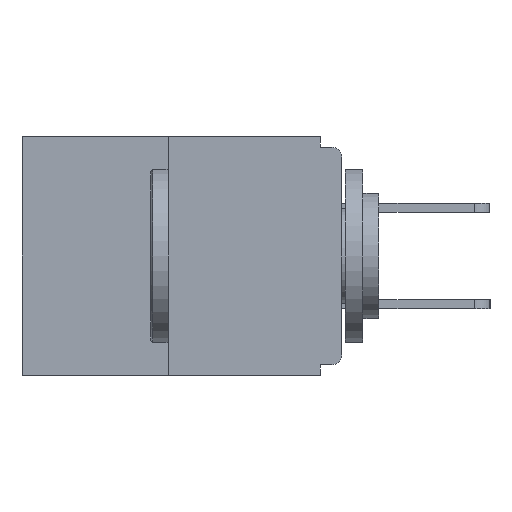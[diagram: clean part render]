
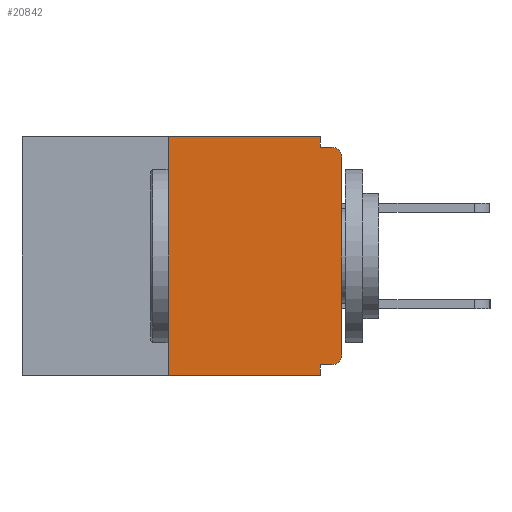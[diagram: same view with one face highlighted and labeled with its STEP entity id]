
A CAD part, left-side view. The second image highlights one B-rep face of the part: STEP entity #20842.
In plain terms, the highlighted planar face has unit normal (-1, 0, 0).
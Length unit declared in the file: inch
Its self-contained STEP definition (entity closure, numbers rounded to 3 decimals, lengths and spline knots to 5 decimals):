
#35 = VERTEX_POINT ( 'NONE', #1568 ) ;
#223 = CARTESIAN_POINT ( 'NONE',  ( 0., 0., 0. ) ) ;
#266 = DIRECTION ( 'NONE',  ( 0., 0., 1. ) ) ;
#528 = VECTOR ( 'NONE', #5872, 39.37008 ) ;
#721 = ORIENTED_EDGE ( 'NONE', *, *, #4216, .T. ) ;
#726 = VECTOR ( 'NONE', #266, 39.37008 ) ;
#1271 = CARTESIAN_POINT ( 'NONE',  ( 0., 0.031, -0.015 ) ) ;
#1568 = CARTESIAN_POINT ( 'NONE',  ( 0., 0.015, -0.015 ) ) ;
#2616 = ORIENTED_EDGE ( 'NONE', *, *, #19204, .T. ) ;
#2681 = EDGE_CURVE ( 'NONE', #5634, #35, #19461, .T. ) ;
#3198 = ORIENTED_EDGE ( 'NONE', *, *, #7958, .F. ) ;
#3575 = VERTEX_POINT ( 'NONE', #24287 ) ;
#4006 = EDGE_LOOP ( 'NONE', ( #14954, #20525, #4340, #3198, #5265, #721, #2616, #23189, #13043, #9560 ) ) ;
#4199 = CARTESIAN_POINT ( 'NONE',  ( 0., 0., -0.015 ) ) ;
#4216 = EDGE_CURVE ( 'NONE', #17066, #3575, #17351, .T. ) ;
#4247 = DIRECTION ( 'NONE',  ( -1., 0., 0. ) ) ;
#4340 = ORIENTED_EDGE ( 'NONE', *, *, #8797, .T. ) ;
#4409 = PLANE ( 'NONE',  #13137 ) ;
#4640 = LINE ( 'NONE', #4199, #528 ) ;
#4915 = CARTESIAN_POINT ( 'NONE',  ( 0., 0.25, 0. ) ) ;
#5029 = LINE ( 'NONE', #8013, #17426 ) ;
#5265 = ORIENTED_EDGE ( 'NONE', *, *, #10138, .F. ) ;
#5357 = LINE ( 'NONE', #17469, #25343 ) ;
#5634 = VERTEX_POINT ( 'NONE', #7228 ) ;
#5655 = VECTOR ( 'NONE', #16438, 39.37008 ) ;
#5872 = DIRECTION ( 'NONE',  ( 0., -1., 0. ) ) ;
#7049 = CARTESIAN_POINT ( 'NONE',  ( 0., 0.031, -0.328 ) ) ;
#7228 = CARTESIAN_POINT ( 'NONE',  ( 0., 0., -0.03 ) ) ;
#7535 = LINE ( 'NONE', #25013, #12930 ) ;
#7699 = CARTESIAN_POINT ( 'NONE',  ( 0., 0.25, -0.343 ) ) ;
#7958 = EDGE_CURVE ( 'NONE', #10662, #8174, #5357, .T. ) ;
#8013 = CARTESIAN_POINT ( 'NONE',  ( 0., 0., -0.328 ) ) ;
#8174 = VERTEX_POINT ( 'NONE', #10585 ) ;
#8677 = DIRECTION ( 'NONE',  ( 0., 0., -1. ) ) ;
#8797 = EDGE_CURVE ( 'NONE', #16553, #8174, #7535, .T. ) ;
#9279 = EDGE_CURVE ( 'NONE', #26026, #16123, #17357, .T. ) ;
#9560 = ORIENTED_EDGE ( 'NONE', *, *, #16487, .F. ) ;
#9629 = AXIS2_PLACEMENT_3D ( 'NONE', #12190, #4247, #18341 ) ;
#9908 = CARTESIAN_POINT ( 'NONE',  ( 0., 0.015, -0.03 ) ) ;
#10138 = EDGE_CURVE ( 'NONE', #17066, #10662, #5029, .T. ) ;
#10179 = DIRECTION ( 'NONE',  ( -1., 0., 0. ) ) ;
#10585 = CARTESIAN_POINT ( 'NONE',  ( 0., 0.031, -0.343 ) ) ;
#10662 = VERTEX_POINT ( 'NONE', #7049 ) ;
#11178 = LINE ( 'NONE', #20848, #24805 ) ;
#11510 = AXIS2_PLACEMENT_3D ( 'NONE', #9908, #10179, #16242 ) ;
#12183 = CARTESIAN_POINT ( 'NONE',  ( 0., 0.46, 0. ) ) ;
#12190 = CARTESIAN_POINT ( 'NONE',  ( 0., 0.015, -0.313 ) ) ;
#12930 = VECTOR ( 'NONE', #16897, 39.37008 ) ;
#13043 = ORIENTED_EDGE ( 'NONE', *, *, #20962, .F. ) ;
#13137 = AXIS2_PLACEMENT_3D ( 'NONE', #12183, #18588, #22471 ) ;
#13470 = DIRECTION ( 'NONE',  ( 0., -1., 0. ) ) ;
#13480 = EDGE_CURVE ( 'NONE', #16553, #26026, #16903, .T. ) ;
#13993 = DIRECTION ( 'NONE',  ( 0., 0., -1. ) ) ;
#14392 = VERTEX_POINT ( 'NONE', #1271 ) ;
#14954 = ORIENTED_EDGE ( 'NONE', *, *, #9279, .F. ) ;
#15310 = CARTESIAN_POINT ( 'NONE',  ( 0., 0.031, 0. ) ) ;
#16123 = VERTEX_POINT ( 'NONE', #15310 ) ;
#16242 = DIRECTION ( 'NONE',  ( 0., 0., -1. ) ) ;
#16438 = DIRECTION ( 'NONE',  ( 0., 0., 1. ) ) ;
#16487 = EDGE_CURVE ( 'NONE', #16123, #14392, #11178, .T. ) ;
#16553 = VERTEX_POINT ( 'NONE', #7699 ) ;
#16698 = FACE_OUTER_BOUND ( 'NONE', #4006, .T. ) ;
#16897 = DIRECTION ( 'NONE',  ( 0., -1., 0. ) ) ;
#16903 = LINE ( 'NONE', #20377, #726 ) ;
#17066 = VERTEX_POINT ( 'NONE', #25762 ) ;
#17351 = CIRCLE ( 'NONE', #9629, 0.015 ) ;
#17357 = LINE ( 'NONE', #25599, #24630 ) ;
#17426 = VECTOR ( 'NONE', #20443, 39.37008 ) ;
#17469 = CARTESIAN_POINT ( 'NONE',  ( 0., 0.031, -0.343 ) ) ;
#18341 = DIRECTION ( 'NONE',  ( 0., 0., -1. ) ) ;
#18588 = DIRECTION ( 'NONE',  ( 1., 0., 0. ) ) ;
#18664 = LINE ( 'NONE', #223, #5655 ) ;
#19204 = EDGE_CURVE ( 'NONE', #3575, #5634, #18664, .T. ) ;
#19461 = CIRCLE ( 'NONE', #11510, 0.015 ) ;
#20377 = CARTESIAN_POINT ( 'NONE',  ( 0., 0.25, 0. ) ) ;
#20443 = DIRECTION ( 'NONE',  ( 0., 1., 0. ) ) ;
#20525 = ORIENTED_EDGE ( 'NONE', *, *, #13480, .F. ) ;
#20842 = ADVANCED_FACE ( 'NONE', ( #16698 ), #4409, .F. ) ;
#20848 = CARTESIAN_POINT ( 'NONE',  ( 0., 0.031, 0. ) ) ;
#20962 = EDGE_CURVE ( 'NONE', #14392, #35, #4640, .T. ) ;
#22471 = DIRECTION ( 'NONE',  ( 0., 0., -1. ) ) ;
#23189 = ORIENTED_EDGE ( 'NONE', *, *, #2681, .T. ) ;
#24287 = CARTESIAN_POINT ( 'NONE',  ( 0., 0., -0.313 ) ) ;
#24630 = VECTOR ( 'NONE', #13470, 39.37008 ) ;
#24805 = VECTOR ( 'NONE', #8677, 39.37008 ) ;
#25013 = CARTESIAN_POINT ( 'NONE',  ( 0., 0.46, -0.343 ) ) ;
#25343 = VECTOR ( 'NONE', #13993, 39.37008 ) ;
#25599 = CARTESIAN_POINT ( 'NONE',  ( 0., 0.46, 0. ) ) ;
#25762 = CARTESIAN_POINT ( 'NONE',  ( 0., 0.015, -0.328 ) ) ;
#26026 = VERTEX_POINT ( 'NONE', #4915 ) ;
